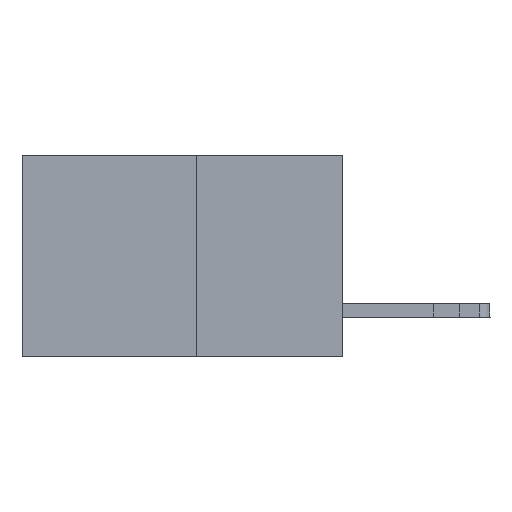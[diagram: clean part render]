
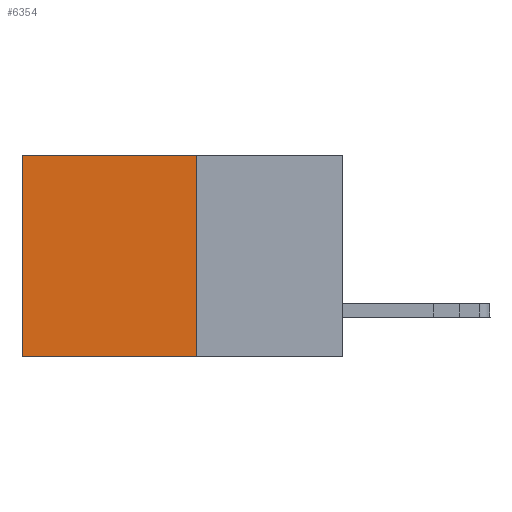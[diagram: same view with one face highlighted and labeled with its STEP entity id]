
A CAD part, left-side view. The second image highlights one B-rep face of the part: STEP entity #6354.
In plain terms, the highlighted planar face has unit normal (-1, 0, 0).
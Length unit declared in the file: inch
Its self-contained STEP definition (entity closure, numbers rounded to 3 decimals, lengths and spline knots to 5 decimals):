
#497 = VECTOR ( 'NONE', #13349, 39.37008 ) ;
#1222 = VERTEX_POINT ( 'NONE', #19929 ) ;
#1390 = DIRECTION ( 'NONE',  ( 1., 0., 0. ) ) ;
#1995 = CARTESIAN_POINT ( 'NONE',  ( 0.277, 0.27, 0. ) ) ;
#4343 = ORIENTED_EDGE ( 'NONE', *, *, #8340, .T. ) ;
#4840 = PLANE ( 'NONE',  #5901 ) ;
#4947 = DIRECTION ( 'NONE',  ( 0., 1., 0. ) ) ;
#5241 = CARTESIAN_POINT ( 'NONE',  ( 0.277, 0.27, -0.37 ) ) ;
#5292 = LINE ( 'NONE', #12326, #5807 ) ;
#5807 = VECTOR ( 'NONE', #4947, 39.37008 ) ;
#5901 = AXIS2_PLACEMENT_3D ( 'NONE', #20390, #1390, #20498 ) ;
#6318 = CARTESIAN_POINT ( 'NONE',  ( 0.277, 0.27, -0.37 ) ) ;
#6354 = ADVANCED_FACE ( 'NONE', ( #7952 ), #4840, .F. ) ;
#6533 = CARTESIAN_POINT ( 'NONE',  ( 0.277, 0.27, 0. ) ) ;
#7232 = EDGE_LOOP ( 'NONE', ( #4343, #18676, #10286, #18713 ) ) ;
#7427 = VECTOR ( 'NONE', #16544, 39.37008 ) ;
#7952 = FACE_OUTER_BOUND ( 'NONE', #7232, .T. ) ;
#7968 = VERTEX_POINT ( 'NONE', #6533 ) ;
#8340 = EDGE_CURVE ( 'NONE', #1222, #20356, #16073, .T. ) ;
#8344 = VECTOR ( 'NONE', #18215, 39.37008 ) ;
#8623 = VERTEX_POINT ( 'NONE', #5241 ) ;
#9331 = EDGE_CURVE ( 'NONE', #7968, #8623, #22206, .T. ) ;
#9393 = CARTESIAN_POINT ( 'NONE',  ( 0.277, 0.59, -0.37 ) ) ;
#10286 = ORIENTED_EDGE ( 'NONE', *, *, #9331, .F. ) ;
#10711 = CARTESIAN_POINT ( 'NONE',  ( 0.277, 0.59, -0.37 ) ) ;
#12326 = CARTESIAN_POINT ( 'NONE',  ( 0.277, 0.27, -0.37 ) ) ;
#13349 = DIRECTION ( 'NONE',  ( 0., 0., -1. ) ) ;
#16073 = LINE ( 'NONE', #9393, #7427 ) ;
#16544 = DIRECTION ( 'NONE',  ( 0., 0., -1. ) ) ;
#18107 = LINE ( 'NONE', #1995, #8344 ) ;
#18215 = DIRECTION ( 'NONE',  ( 0., 1., 0. ) ) ;
#18676 = ORIENTED_EDGE ( 'NONE', *, *, #20152, .F. ) ;
#18713 = ORIENTED_EDGE ( 'NONE', *, *, #18717, .T. ) ;
#18717 = EDGE_CURVE ( 'NONE', #7968, #1222, #18107, .T. ) ;
#19929 = CARTESIAN_POINT ( 'NONE',  ( 0.277, 0.59, 0. ) ) ;
#20152 = EDGE_CURVE ( 'NONE', #8623, #20356, #5292, .T. ) ;
#20356 = VERTEX_POINT ( 'NONE', #10711 ) ;
#20390 = CARTESIAN_POINT ( 'NONE',  ( 0.277, 0.27, -0.37 ) ) ;
#20498 = DIRECTION ( 'NONE',  ( 0., 0., -1. ) ) ;
#22206 = LINE ( 'NONE', #6318, #497 ) ;
